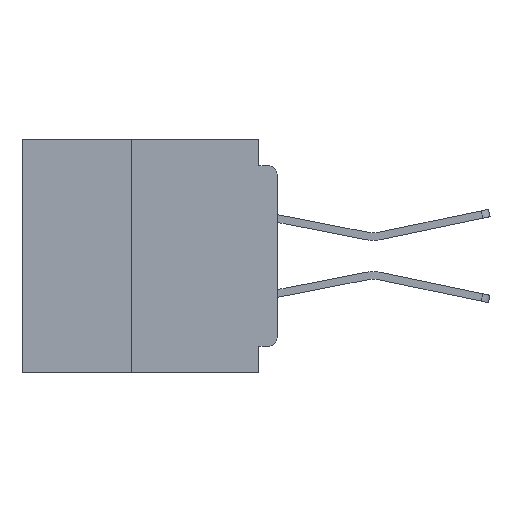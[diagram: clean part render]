
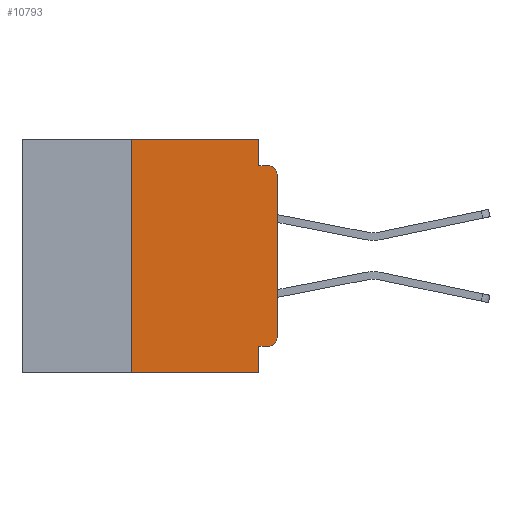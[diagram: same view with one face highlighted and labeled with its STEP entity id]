
A CAD part, left-side view. The second image highlights one B-rep face of the part: STEP entity #10793.
In plain terms, the highlighted planar face has unit normal (-1, 0, 0).
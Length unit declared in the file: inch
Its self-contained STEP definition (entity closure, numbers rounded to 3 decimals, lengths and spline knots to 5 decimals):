
#284 = CARTESIAN_POINT ( 'NONE',  ( 0., 0., -0.34 ) ) ;
#1649 = EDGE_CURVE ( 'NONE', #47926, #2118, #13569, .T. ) ;
#1742 = DIRECTION ( 'NONE',  ( 0., -1., 0. ) ) ;
#2118 = VERTEX_POINT ( 'NONE', #27114 ) ;
#2739 = ORIENTED_EDGE ( 'NONE', *, *, #15831, .F. ) ;
#3439 = AXIS2_PLACEMENT_3D ( 'NONE', #34292, #12025, #38014 ) ;
#3533 = FACE_OUTER_BOUND ( 'NONE', #9240, .T. ) ;
#3632 = VECTOR ( 'NONE', #21351, 39.37008 ) ;
#5098 = EDGE_CURVE ( 'NONE', #9265, #42903, #17820, .T. ) ;
#5109 = ORIENTED_EDGE ( 'NONE', *, *, #1649, .F. ) ;
#5944 = CARTESIAN_POINT ( 'NONE',  ( 0., 0., -0.06 ) ) ;
#6230 = CARTESIAN_POINT ( 'NONE',  ( 0., 0.031, 0. ) ) ;
#6623 = LINE ( 'NONE', #47115, #15384 ) ;
#6665 = EDGE_CURVE ( 'NONE', #32625, #42903, #36872, .T. ) ;
#9141 = DIRECTION ( 'NONE',  ( 0., 0., -1. ) ) ;
#9189 = ORIENTED_EDGE ( 'NONE', *, *, #21167, .F. ) ;
#9240 = EDGE_LOOP ( 'NONE', ( #13248, #15588, #45151, #47449, #9189, #19060, #31297, #2739, #5109, #15031 ) ) ;
#9265 = VERTEX_POINT ( 'NONE', #28393 ) ;
#9584 = DIRECTION ( 'NONE',  ( 0., 0., -1. ) ) ;
#10144 = CARTESIAN_POINT ( 'NONE',  ( 0., 0.25, -0.4 ) ) ;
#10793 = ADVANCED_FACE ( 'NONE', ( #3533 ), #27658, .F. ) ;
#12025 = DIRECTION ( 'NONE',  ( -1., 0., 0. ) ) ;
#12154 = VERTEX_POINT ( 'NONE', #6230 ) ;
#13248 = ORIENTED_EDGE ( 'NONE', *, *, #35957, .T. ) ;
#13330 = EDGE_CURVE ( 'NONE', #31390, #30164, #16193, .T. ) ;
#13373 = DIRECTION ( 'NONE',  ( -1., 0., 0. ) ) ;
#13401 = DIRECTION ( 'NONE',  ( 0., -1., 0. ) ) ;
#13569 = LINE ( 'NONE', #27810, #42028 ) ;
#15031 = ORIENTED_EDGE ( 'NONE', *, *, #34100, .T. ) ;
#15384 = VECTOR ( 'NONE', #21252, 39.37008 ) ;
#15588 = ORIENTED_EDGE ( 'NONE', *, *, #6665, .T. ) ;
#15831 = EDGE_CURVE ( 'NONE', #2118, #30164, #28891, .T. ) ;
#16193 = LINE ( 'NONE', #16604, #34804 ) ;
#16410 = CARTESIAN_POINT ( 'NONE',  ( 0., 0.031, -0.4 ) ) ;
#16604 = CARTESIAN_POINT ( 'NONE',  ( 0., 0.437, -0.4 ) ) ;
#17533 = DIRECTION ( 'NONE',  ( 0., -1., 0. ) ) ;
#17706 = LINE ( 'NONE', #20869, #26454 ) ;
#17820 = LINE ( 'NONE', #36087, #38752 ) ;
#18816 = CARTESIAN_POINT ( 'NONE',  ( 0., 0.015, -0.355 ) ) ;
#18999 = VECTOR ( 'NONE', #31342, 39.37008 ) ;
#19060 = ORIENTED_EDGE ( 'NONE', *, *, #41631, .F. ) ;
#19794 = LINE ( 'NONE', #46680, #20966 ) ;
#20029 = CARTESIAN_POINT ( 'NONE',  ( 0., 0.437, 0. ) ) ;
#20420 = AXIS2_PLACEMENT_3D ( 'NONE', #35634, #13373, #39331 ) ;
#20869 = CARTESIAN_POINT ( 'NONE',  ( 0., 0.437, 0. ) ) ;
#20966 = VECTOR ( 'NONE', #9584, 39.37008 ) ;
#21167 = EDGE_CURVE ( 'NONE', #38941, #12154, #17706, .T. ) ;
#21252 = DIRECTION ( 'NONE',  ( 0., 0., 1. ) ) ;
#21351 = DIRECTION ( 'NONE',  ( 0., 0., 1. ) ) ;
#26454 = VECTOR ( 'NONE', #13401, 39.37008 ) ;
#27114 = CARTESIAN_POINT ( 'NONE',  ( 0., 0.031, -0.355 ) ) ;
#27658 = PLANE ( 'NONE',  #29904 ) ;
#27810 = CARTESIAN_POINT ( 'NONE',  ( 0., 0., -0.355 ) ) ;
#28136 = DIRECTION ( 'NONE',  ( 0., 1., 0. ) ) ;
#28393 = CARTESIAN_POINT ( 'NONE',  ( 0., 0.031, -0.045 ) ) ;
#28891 = LINE ( 'NONE', #16410, #18999 ) ;
#29196 = EDGE_CURVE ( 'NONE', #12154, #9265, #19794, .T. ) ;
#29904 = AXIS2_PLACEMENT_3D ( 'NONE', #20029, #31408, #9141 ) ;
#30164 = VERTEX_POINT ( 'NONE', #46552 ) ;
#31297 = ORIENTED_EDGE ( 'NONE', *, *, #13330, .T. ) ;
#31342 = DIRECTION ( 'NONE',  ( 0., 0., -1. ) ) ;
#31390 = VERTEX_POINT ( 'NONE', #39044 ) ;
#31408 = DIRECTION ( 'NONE',  ( 1., 0., 0. ) ) ;
#32428 = CIRCLE ( 'NONE', #3439, 0.015 ) ;
#32625 = VERTEX_POINT ( 'NONE', #5944 ) ;
#33416 = CARTESIAN_POINT ( 'NONE',  ( 0., 0.015, -0.045 ) ) ;
#34100 = EDGE_CURVE ( 'NONE', #47926, #43642, #32428, .T. ) ;
#34292 = CARTESIAN_POINT ( 'NONE',  ( 0., 0.015, -0.34 ) ) ;
#34804 = VECTOR ( 'NONE', #1742, 39.37008 ) ;
#35634 = CARTESIAN_POINT ( 'NONE',  ( 0., 0.015, -0.06 ) ) ;
#35957 = EDGE_CURVE ( 'NONE', #43642, #32625, #6623, .T. ) ;
#36087 = CARTESIAN_POINT ( 'NONE',  ( 0., 0., -0.045 ) ) ;
#36832 = CARTESIAN_POINT ( 'NONE',  ( 0., 0.25, 0. ) ) ;
#36872 = CIRCLE ( 'NONE', #20420, 0.015 ) ;
#38014 = DIRECTION ( 'NONE',  ( 0., 0., -1. ) ) ;
#38752 = VECTOR ( 'NONE', #17533, 39.37008 ) ;
#38941 = VERTEX_POINT ( 'NONE', #36832 ) ;
#39044 = CARTESIAN_POINT ( 'NONE',  ( 0., 0.25, -0.4 ) ) ;
#39331 = DIRECTION ( 'NONE',  ( 0., 0., -1. ) ) ;
#41631 = EDGE_CURVE ( 'NONE', #31390, #38941, #42032, .T. ) ;
#42028 = VECTOR ( 'NONE', #28136, 39.37008 ) ;
#42032 = LINE ( 'NONE', #10144, #3632 ) ;
#42903 = VERTEX_POINT ( 'NONE', #33416 ) ;
#43642 = VERTEX_POINT ( 'NONE', #284 ) ;
#45151 = ORIENTED_EDGE ( 'NONE', *, *, #5098, .F. ) ;
#46552 = CARTESIAN_POINT ( 'NONE',  ( 0., 0.031, -0.4 ) ) ;
#46680 = CARTESIAN_POINT ( 'NONE',  ( 0., 0.031, 0. ) ) ;
#47115 = CARTESIAN_POINT ( 'NONE',  ( 0., 0., 0. ) ) ;
#47449 = ORIENTED_EDGE ( 'NONE', *, *, #29196, .F. ) ;
#47926 = VERTEX_POINT ( 'NONE', #18816 ) ;
